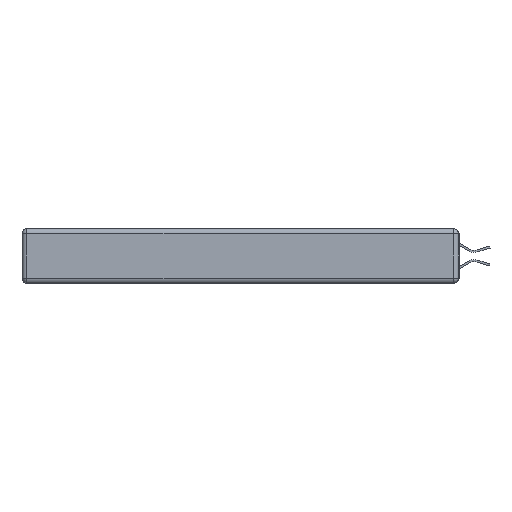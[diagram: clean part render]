
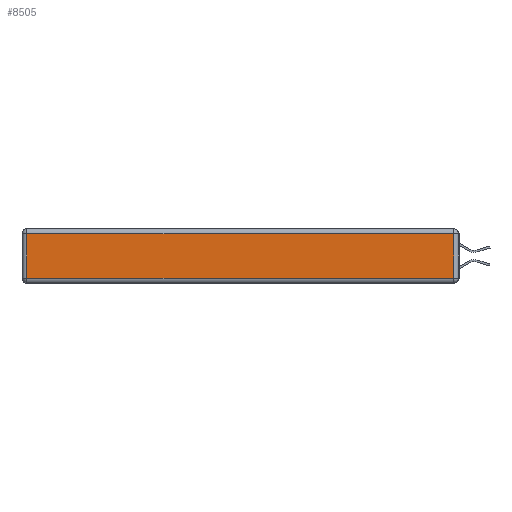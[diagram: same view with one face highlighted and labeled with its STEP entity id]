
A CAD part, left-side view. The second image highlights one B-rep face of the part: STEP entity #8505.
In plain terms, the highlighted planar face has unit normal (-1, 0, 0).
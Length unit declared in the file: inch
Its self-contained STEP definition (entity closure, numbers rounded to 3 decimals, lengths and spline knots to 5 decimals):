
#439 = CARTESIAN_POINT ( 'NONE',  ( 0., 0.03, -0.03 ) ) ;
#1176 = DIRECTION ( 'NONE',  ( 0., 0., -1. ) ) ;
#2112 = CARTESIAN_POINT ( 'NONE',  ( 0., 2.72, -0.03 ) ) ;
#2246 = VERTEX_POINT ( 'NONE', #2112 ) ;
#2611 = DIRECTION ( 'NONE',  ( 0., 1., 0. ) ) ;
#2704 = EDGE_LOOP ( 'NONE', ( #13637, #4212, #13675, #6796 ) ) ;
#3896 = VECTOR ( 'NONE', #2611, 39.37008 ) ;
#3994 = LINE ( 'NONE', #15121, #11884 ) ;
#4212 = ORIENTED_EDGE ( 'NONE', *, *, #11801, .T. ) ;
#4275 = LINE ( 'NONE', #18006, #17749 ) ;
#5412 = LINE ( 'NONE', #16328, #3896 ) ;
#5571 = DIRECTION ( 'NONE',  ( 0., 0., 1. ) ) ;
#6290 = VECTOR ( 'NONE', #9960, 39.37008 ) ;
#6661 = CARTESIAN_POINT ( 'NONE',  ( 0., 2.72, -0.313 ) ) ;
#6796 = ORIENTED_EDGE ( 'NONE', *, *, #18005, .T. ) ;
#7266 = CARTESIAN_POINT ( 'NONE',  ( 0., 0.03, -0.343 ) ) ;
#8505 = ADVANCED_FACE ( 'NONE', ( #12986 ), #11831, .T. ) ;
#9281 = DIRECTION ( 'NONE',  ( -1., 0., 0. ) ) ;
#9960 = DIRECTION ( 'NONE',  ( 0., 0., 1. ) ) ;
#10016 = LINE ( 'NONE', #7266, #6290 ) ;
#10732 = AXIS2_PLACEMENT_3D ( 'NONE', #15142, #9281, #5571 ) ;
#11801 = EDGE_CURVE ( 'NONE', #13571, #15188, #10016, .T. ) ;
#11831 = PLANE ( 'NONE',  #10732 ) ;
#11884 = VECTOR ( 'NONE', #1176, 39.37008 ) ;
#12986 = FACE_OUTER_BOUND ( 'NONE', #2704, .T. ) ;
#13571 = VERTEX_POINT ( 'NONE', #14108 ) ;
#13637 = ORIENTED_EDGE ( 'NONE', *, *, #16811, .T. ) ;
#13675 = ORIENTED_EDGE ( 'NONE', *, *, #15448, .T. ) ;
#13796 = DIRECTION ( 'NONE',  ( 0., -1., 0. ) ) ;
#14108 = CARTESIAN_POINT ( 'NONE',  ( 0., 0.03, -0.313 ) ) ;
#15121 = CARTESIAN_POINT ( 'NONE',  ( 0., 2.72, -0.343 ) ) ;
#15142 = CARTESIAN_POINT ( 'NONE',  ( 0., 0., -0.343 ) ) ;
#15188 = VERTEX_POINT ( 'NONE', #439 ) ;
#15448 = EDGE_CURVE ( 'NONE', #15188, #2246, #5412, .T. ) ;
#16328 = CARTESIAN_POINT ( 'NONE',  ( 0., 2.75, -0.03 ) ) ;
#16811 = EDGE_CURVE ( 'NONE', #17947, #13571, #4275, .T. ) ;
#17749 = VECTOR ( 'NONE', #13796, 39.37008 ) ;
#17947 = VERTEX_POINT ( 'NONE', #6661 ) ;
#18005 = EDGE_CURVE ( 'NONE', #2246, #17947, #3994, .T. ) ;
#18006 = CARTESIAN_POINT ( 'NONE',  ( 0., 0., -0.313 ) ) ;
